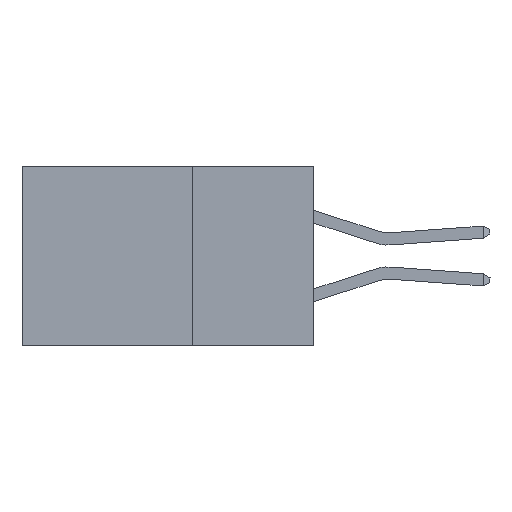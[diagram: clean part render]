
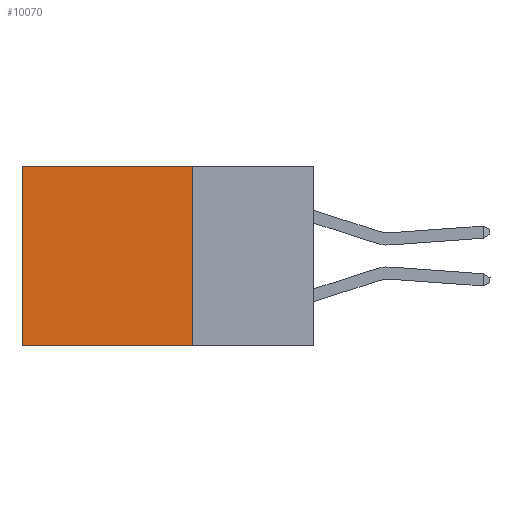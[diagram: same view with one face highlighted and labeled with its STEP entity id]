
A CAD part, left-side view. The second image highlights one B-rep face of the part: STEP entity #10070.
In plain terms, the highlighted planar face has unit normal (-1, 0, 0).
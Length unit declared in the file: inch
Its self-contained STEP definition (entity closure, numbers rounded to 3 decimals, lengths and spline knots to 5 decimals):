
#178 = VERTEX_POINT ( 'NONE', #13399 ) ;
#256 = LINE ( 'NONE', #3944, #3816 ) ;
#943 = PLANE ( 'NONE',  #4401 ) ;
#1939 = EDGE_LOOP ( 'NONE', ( #20234, #3316, #20545, #23599 ) ) ;
#1944 = DIRECTION ( 'NONE',  ( 0., 1., 0. ) ) ;
#3316 = ORIENTED_EDGE ( 'NONE', *, *, #18750, .F. ) ;
#3462 = VECTOR ( 'NONE', #7394, 39.37008 ) ;
#3816 = VECTOR ( 'NONE', #1944, 39.37008 ) ;
#3944 = CARTESIAN_POINT ( 'NONE',  ( 0.2875, 0.25, -0.37 ) ) ;
#4401 = AXIS2_PLACEMENT_3D ( 'NONE', #16207, #8680, #21936 ) ;
#7291 = VERTEX_POINT ( 'NONE', #10235 ) ;
#7394 = DIRECTION ( 'NONE',  ( 0., 0., -1. ) ) ;
#8478 = CARTESIAN_POINT ( 'NONE',  ( 0.2875, 0.6, 0. ) ) ;
#8680 = DIRECTION ( 'NONE',  ( 1., 0., 0. ) ) ;
#9042 = CARTESIAN_POINT ( 'NONE',  ( 0.2875, 0.6, -0.37 ) ) ;
#9452 = VECTOR ( 'NONE', #10446, 39.37008 ) ;
#10070 = ADVANCED_FACE ( 'NONE', ( #12027 ), #943, .F. ) ;
#10235 = CARTESIAN_POINT ( 'NONE',  ( 0.2875, 0.25, 0. ) ) ;
#10446 = DIRECTION ( 'NONE',  ( 0., 1., 0. ) ) ;
#10629 = VECTOR ( 'NONE', #16704, 39.37008 ) ;
#11217 = LINE ( 'NONE', #16380, #10629 ) ;
#12027 = FACE_OUTER_BOUND ( 'NONE', #1939, .T. ) ;
#13399 = CARTESIAN_POINT ( 'NONE',  ( 0.2875, 0.25, -0.37 ) ) ;
#15369 = LINE ( 'NONE', #19871, #9452 ) ;
#16207 = CARTESIAN_POINT ( 'NONE',  ( 0.2875, 0.25, 0. ) ) ;
#16380 = CARTESIAN_POINT ( 'NONE',  ( 0.2875, 0.25, 0. ) ) ;
#16474 = LINE ( 'NONE', #22478, #3462 ) ;
#16704 = DIRECTION ( 'NONE',  ( 0., 0., -1. ) ) ;
#17135 = EDGE_CURVE ( 'NONE', #7291, #24425, #15369, .T. ) ;
#18336 = VERTEX_POINT ( 'NONE', #9042 ) ;
#18750 = EDGE_CURVE ( 'NONE', #178, #18336, #256, .T. ) ;
#19871 = CARTESIAN_POINT ( 'NONE',  ( 0.2875, 0.25, 0. ) ) ;
#20234 = ORIENTED_EDGE ( 'NONE', *, *, #22121, .T. ) ;
#20545 = ORIENTED_EDGE ( 'NONE', *, *, #21217, .F. ) ;
#21217 = EDGE_CURVE ( 'NONE', #7291, #178, #11217, .T. ) ;
#21936 = DIRECTION ( 'NONE',  ( 0., 0., -1. ) ) ;
#22121 = EDGE_CURVE ( 'NONE', #24425, #18336, #16474, .T. ) ;
#22478 = CARTESIAN_POINT ( 'NONE',  ( 0.2875, 0.6, 0. ) ) ;
#23599 = ORIENTED_EDGE ( 'NONE', *, *, #17135, .T. ) ;
#24425 = VERTEX_POINT ( 'NONE', #8478 ) ;
